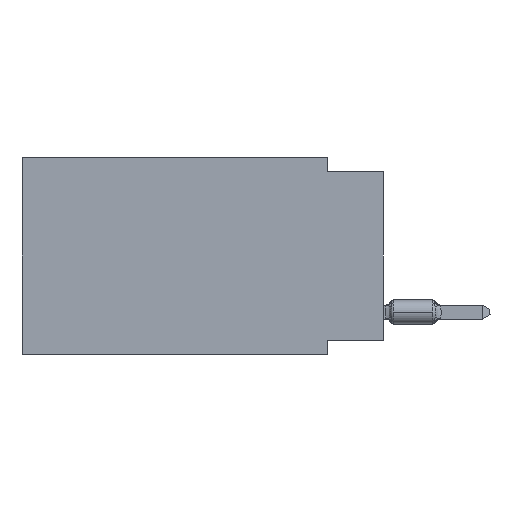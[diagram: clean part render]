
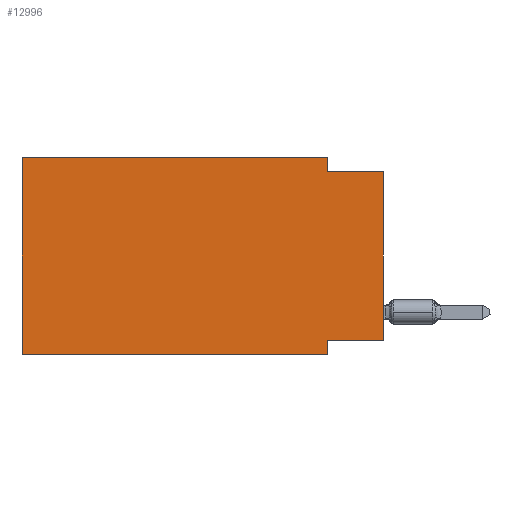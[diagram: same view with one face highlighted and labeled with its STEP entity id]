
A CAD part, left-side view. The second image highlights one B-rep face of the part: STEP entity #12996.
In plain terms, the highlighted planar face has unit normal (-1, 0, 0).
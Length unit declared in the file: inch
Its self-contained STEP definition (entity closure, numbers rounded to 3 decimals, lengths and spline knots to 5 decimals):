
#652 = ORIENTED_EDGE ( 'NONE', *, *, #22070, .T. ) ;
#769 = VECTOR ( 'NONE', #20440, 39.37008 ) ;
#1785 = EDGE_CURVE ( 'NONE', #2472, #6429, #31010, .T. ) ;
#2238 = DIRECTION ( 'NONE',  ( 0., -1., 0. ) ) ;
#2472 = VERTEX_POINT ( 'NONE', #31168 ) ;
#2548 = EDGE_CURVE ( 'NONE', #18412, #15948, #3964, .T. ) ;
#3615 = VERTEX_POINT ( 'NONE', #13191 ) ;
#3964 = LINE ( 'NONE', #30534, #27268 ) ;
#5299 = EDGE_CURVE ( 'NONE', #29569, #29401, #19980, .T. ) ;
#5433 = LINE ( 'NONE', #25179, #29632 ) ;
#6429 = VERTEX_POINT ( 'NONE', #25178 ) ;
#6873 = VECTOR ( 'NONE', #20314, 39.37008 ) ;
#7072 = EDGE_LOOP ( 'NONE', ( #31924, #30320, #12828, #20932, #10685, #652, #8217, #27572 ) ) ;
#7685 = CARTESIAN_POINT ( 'NONE',  ( 0., 0., -0.325 ) ) ;
#7834 = LINE ( 'NONE', #10418, #769 ) ;
#8217 = ORIENTED_EDGE ( 'NONE', *, *, #5299, .F. ) ;
#8822 = CARTESIAN_POINT ( 'NONE',  ( 0., 0.645, 0. ) ) ;
#9017 = EDGE_CURVE ( 'NONE', #3615, #15948, #18313, .T. ) ;
#10418 = CARTESIAN_POINT ( 'NONE',  ( 0., 0.645, 0. ) ) ;
#10685 = ORIENTED_EDGE ( 'NONE', *, *, #13428, .F. ) ;
#10801 = EDGE_CURVE ( 'NONE', #6429, #3615, #5433, .T. ) ;
#11021 = DIRECTION ( 'NONE',  ( 0., -1., 0. ) ) ;
#12252 = VECTOR ( 'NONE', #2238, 39.37008 ) ;
#12281 = FACE_OUTER_BOUND ( 'NONE', #7072, .T. ) ;
#12635 = AXIS2_PLACEMENT_3D ( 'NONE', #20039, #17297, #26865 ) ;
#12827 = CARTESIAN_POINT ( 'NONE',  ( 0., 0.1, -0.35 ) ) ;
#12828 = ORIENTED_EDGE ( 'NONE', *, *, #10801, .F. ) ;
#12996 = ADVANCED_FACE ( 'NONE', ( #12281 ), #27502, .F. ) ;
#13023 = CARTESIAN_POINT ( 'NONE',  ( 0., 0.1, -0.35 ) ) ;
#13191 = CARTESIAN_POINT ( 'NONE',  ( 0., 0.1, -0.025 ) ) ;
#13428 = EDGE_CURVE ( 'NONE', #22341, #2472, #7834, .T. ) ;
#13672 = DIRECTION ( 'NONE',  ( 0., 0., 1. ) ) ;
#14230 = LINE ( 'NONE', #19721, #12252 ) ;
#15948 = VERTEX_POINT ( 'NONE', #31813 ) ;
#16332 = CARTESIAN_POINT ( 'NONE',  ( 0., 0.1, -0.325 ) ) ;
#17078 = VECTOR ( 'NONE', #18203, 39.37008 ) ;
#17297 = DIRECTION ( 'NONE',  ( 1., 0., 0. ) ) ;
#18203 = DIRECTION ( 'NONE',  ( 0., 1., 0. ) ) ;
#18313 = LINE ( 'NONE', #30793, #25942 ) ;
#18412 = VERTEX_POINT ( 'NONE', #23406 ) ;
#19721 = CARTESIAN_POINT ( 'NONE',  ( 0., 0.645, -0.35 ) ) ;
#19980 = LINE ( 'NONE', #13023, #6873 ) ;
#20039 = CARTESIAN_POINT ( 'NONE',  ( 0., 0.645, 0. ) ) ;
#20314 = DIRECTION ( 'NONE',  ( 0., 0., -1. ) ) ;
#20440 = DIRECTION ( 'NONE',  ( 0., 0., 1. ) ) ;
#20463 = DIRECTION ( 'NONE',  ( 0., 0., -1. ) ) ;
#20932 = ORIENTED_EDGE ( 'NONE', *, *, #1785, .F. ) ;
#22070 = EDGE_CURVE ( 'NONE', #22341, #29401, #14230, .T. ) ;
#22341 = VERTEX_POINT ( 'NONE', #28284 ) ;
#23406 = CARTESIAN_POINT ( 'NONE',  ( 0., 0., -0.325 ) ) ;
#23710 = DIRECTION ( 'NONE',  ( 0., -1., 0. ) ) ;
#24496 = VECTOR ( 'NONE', #23710, 39.37008 ) ;
#25178 = CARTESIAN_POINT ( 'NONE',  ( 0., 0.1, 0. ) ) ;
#25179 = CARTESIAN_POINT ( 'NONE',  ( 0., 0.1, 0. ) ) ;
#25942 = VECTOR ( 'NONE', #11021, 39.37008 ) ;
#26865 = DIRECTION ( 'NONE',  ( 0., 0., -1. ) ) ;
#27268 = VECTOR ( 'NONE', #13672, 39.37008 ) ;
#27502 = PLANE ( 'NONE',  #12635 ) ;
#27572 = ORIENTED_EDGE ( 'NONE', *, *, #30158, .F. ) ;
#28284 = CARTESIAN_POINT ( 'NONE',  ( 0., 0.645, -0.35 ) ) ;
#29401 = VERTEX_POINT ( 'NONE', #12827 ) ;
#29569 = VERTEX_POINT ( 'NONE', #16332 ) ;
#29632 = VECTOR ( 'NONE', #20463, 39.37008 ) ;
#29879 = LINE ( 'NONE', #7685, #17078 ) ;
#30158 = EDGE_CURVE ( 'NONE', #18412, #29569, #29879, .T. ) ;
#30320 = ORIENTED_EDGE ( 'NONE', *, *, #9017, .F. ) ;
#30534 = CARTESIAN_POINT ( 'NONE',  ( 0., 0., 0. ) ) ;
#30793 = CARTESIAN_POINT ( 'NONE',  ( 0., 0., -0.025 ) ) ;
#31010 = LINE ( 'NONE', #8822, #24496 ) ;
#31168 = CARTESIAN_POINT ( 'NONE',  ( 0., 0.645, 0. ) ) ;
#31813 = CARTESIAN_POINT ( 'NONE',  ( 0., 0., -0.025 ) ) ;
#31924 = ORIENTED_EDGE ( 'NONE', *, *, #2548, .T. ) ;
